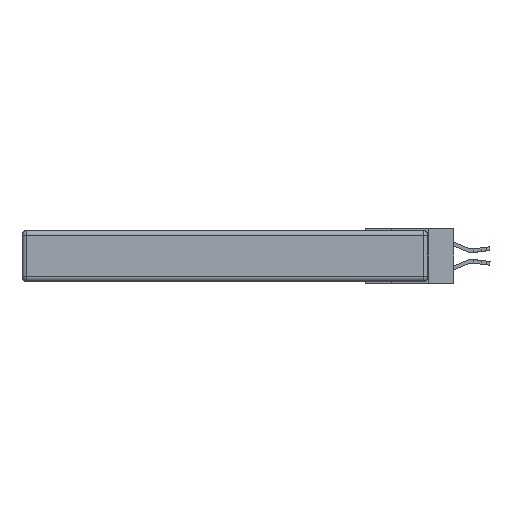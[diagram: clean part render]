
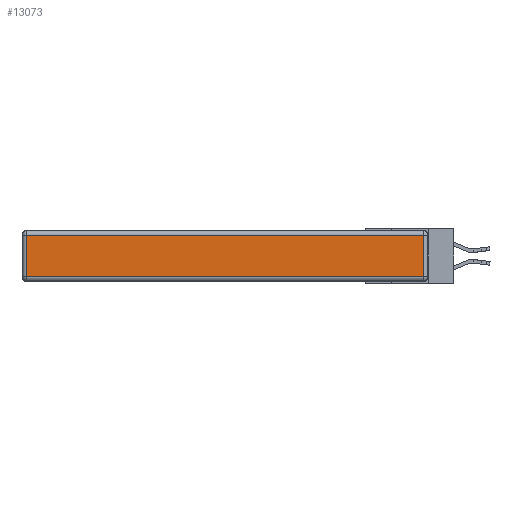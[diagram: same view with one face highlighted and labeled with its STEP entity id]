
A CAD part, left-side view. The second image highlights one B-rep face of the part: STEP entity #13073.
In plain terms, the highlighted planar face has unit normal (-1, 0, 0).
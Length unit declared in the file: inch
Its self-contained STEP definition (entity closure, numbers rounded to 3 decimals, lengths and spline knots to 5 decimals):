
#73 = PLANE ( 'NONE',  #10052 ) ;
#199 = DIRECTION ( 'NONE',  ( 0., 0., 1. ) ) ;
#1333 = CARTESIAN_POINT ( 'NONE',  ( 0., 0.03, -0.03 ) ) ;
#2101 = FACE_OUTER_BOUND ( 'NONE', #15378, .T. ) ;
#2169 = LINE ( 'NONE', #8862, #11779 ) ;
#3403 = VECTOR ( 'NONE', #3999, 39.37008 ) ;
#3999 = DIRECTION ( 'NONE',  ( 0., 0., 1. ) ) ;
#5049 = VECTOR ( 'NONE', #16895, 39.37008 ) ;
#6063 = VECTOR ( 'NONE', #14660, 39.37008 ) ;
#6093 = DIRECTION ( 'NONE',  ( -1., 0., 0. ) ) ;
#6161 = CARTESIAN_POINT ( 'NONE',  ( 0., 2.72, -0.313 ) ) ;
#6712 = VERTEX_POINT ( 'NONE', #18322 ) ;
#7968 = VERTEX_POINT ( 'NONE', #1333 ) ;
#8439 = EDGE_CURVE ( 'NONE', #13784, #6712, #17432, .T. ) ;
#8788 = CARTESIAN_POINT ( 'NONE',  ( 0., 2.72, -0.03 ) ) ;
#8862 = CARTESIAN_POINT ( 'NONE',  ( 0., 2.75, -0.03 ) ) ;
#9014 = CARTESIAN_POINT ( 'NONE',  ( 0., 0., -0.343 ) ) ;
#9059 = DIRECTION ( 'NONE',  ( 0., 1., 0. ) ) ;
#10052 = AXIS2_PLACEMENT_3D ( 'NONE', #9014, #6093, #199 ) ;
#10522 = ORIENTED_EDGE ( 'NONE', *, *, #17646, .T. ) ;
#11677 = CARTESIAN_POINT ( 'NONE',  ( 0., 2.72, -0.343 ) ) ;
#11779 = VECTOR ( 'NONE', #9059, 39.37008 ) ;
#12154 = VERTEX_POINT ( 'NONE', #8788 ) ;
#12584 = ORIENTED_EDGE ( 'NONE', *, *, #15338, .T. ) ;
#12907 = ORIENTED_EDGE ( 'NONE', *, *, #16722, .T. ) ;
#13018 = CARTESIAN_POINT ( 'NONE',  ( 0., 0.03, -0.343 ) ) ;
#13073 = ADVANCED_FACE ( 'NONE', ( #2101 ), #73, .T. ) ;
#13784 = VERTEX_POINT ( 'NONE', #6161 ) ;
#14660 = DIRECTION ( 'NONE',  ( 0., 0., -1. ) ) ;
#15338 = EDGE_CURVE ( 'NONE', #6712, #7968, #17408, .T. ) ;
#15378 = EDGE_LOOP ( 'NONE', ( #18842, #12584, #12907, #10522 ) ) ;
#15475 = LINE ( 'NONE', #11677, #6063 ) ;
#16722 = EDGE_CURVE ( 'NONE', #7968, #12154, #2169, .T. ) ;
#16895 = DIRECTION ( 'NONE',  ( 0., -1., 0. ) ) ;
#17408 = LINE ( 'NONE', #13018, #3403 ) ;
#17432 = LINE ( 'NONE', #18285, #5049 ) ;
#17646 = EDGE_CURVE ( 'NONE', #12154, #13784, #15475, .T. ) ;
#18285 = CARTESIAN_POINT ( 'NONE',  ( 0., 0., -0.313 ) ) ;
#18322 = CARTESIAN_POINT ( 'NONE',  ( 0., 0.03, -0.313 ) ) ;
#18842 = ORIENTED_EDGE ( 'NONE', *, *, #8439, .T. ) ;
